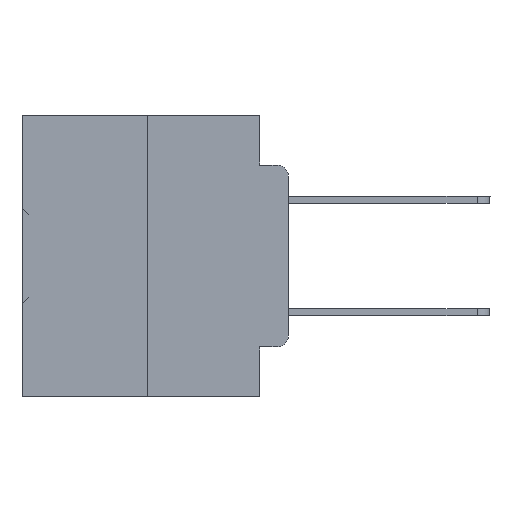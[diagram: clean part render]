
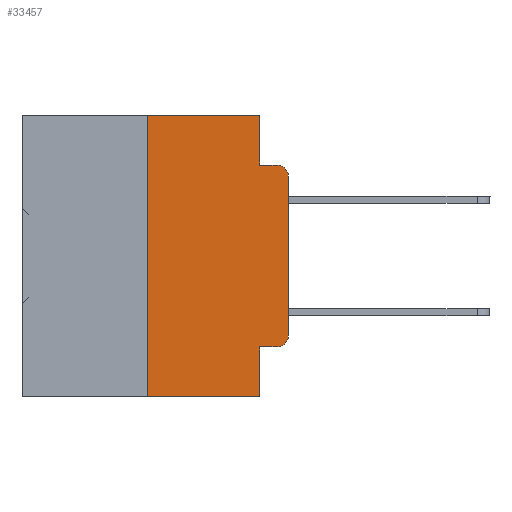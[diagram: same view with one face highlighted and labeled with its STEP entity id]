
A CAD part, left-side view. The second image highlights one B-rep face of the part: STEP entity #33457.
In plain terms, the highlighted planar face has unit normal (-1, 0, 0).
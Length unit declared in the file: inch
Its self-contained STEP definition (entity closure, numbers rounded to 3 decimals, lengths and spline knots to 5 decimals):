
#88 = CARTESIAN_POINT ( 'NONE',  ( 0., 0.02, -0.3915 ) ) ;
#1342 = ORIENTED_EDGE ( 'NONE', *, *, #35961, .T. ) ;
#1684 = CIRCLE ( 'NONE', #11143, 0.02 ) ;
#2079 = ORIENTED_EDGE ( 'NONE', *, *, #12284, .F. ) ;
#2376 = DIRECTION ( 'NONE',  ( 0., 0., 1. ) ) ;
#2978 = ORIENTED_EDGE ( 'NONE', *, *, #35231, .T. ) ;
#3258 = DIRECTION ( 'NONE',  ( 0., -1., 0. ) ) ;
#3757 = ORIENTED_EDGE ( 'NONE', *, *, #28549, .T. ) ;
#3790 = CARTESIAN_POINT ( 'NONE',  ( 0., 0.02, -0.1085 ) ) ;
#4803 = VECTOR ( 'NONE', #38339, 39.37008 ) ;
#5475 = CARTESIAN_POINT ( 'NONE',  ( 0., 0.051, 0. ) ) ;
#5588 = VERTEX_POINT ( 'NONE', #29817 ) ;
#5897 = VERTEX_POINT ( 'NONE', #31747 ) ;
#6473 = EDGE_CURVE ( 'NONE', #5588, #16402, #15289, .T. ) ;
#6574 = VERTEX_POINT ( 'NONE', #9581 ) ;
#6600 = LINE ( 'NONE', #30233, #21007 ) ;
#6768 = CARTESIAN_POINT ( 'NONE',  ( 0., 0.25, 0. ) ) ;
#6769 = VECTOR ( 'NONE', #21133, 39.37008 ) ;
#7254 = AXIS2_PLACEMENT_3D ( 'NONE', #20792, #32813, #12151 ) ;
#8022 = VECTOR ( 'NONE', #2376, 39.37008 ) ;
#8224 = VERTEX_POINT ( 'NONE', #24712 ) ;
#9144 = CARTESIAN_POINT ( 'NONE',  ( 0., 0.051, -0.4115 ) ) ;
#9257 = LINE ( 'NONE', #21049, #28748 ) ;
#9489 = DIRECTION ( 'NONE',  ( 0., 0., -1. ) ) ;
#9581 = CARTESIAN_POINT ( 'NONE',  ( 0., 0.02, -0.4115 ) ) ;
#9919 = LINE ( 'NONE', #6768, #32879 ) ;
#11143 = AXIS2_PLACEMENT_3D ( 'NONE', #3790, #12254, #9489 ) ;
#11193 = EDGE_CURVE ( 'NONE', #8224, #28474, #9919, .T. ) ;
#11759 = LINE ( 'NONE', #5475, #17265 ) ;
#12151 = DIRECTION ( 'NONE',  ( 0., 0., -1. ) ) ;
#12228 = ORIENTED_EDGE ( 'NONE', *, *, #6473, .F. ) ;
#12254 = DIRECTION ( 'NONE',  ( -1., 0., 0. ) ) ;
#12284 = EDGE_CURVE ( 'NONE', #23828, #20563, #11759, .T. ) ;
#12286 = DIRECTION ( 'NONE',  ( -1., 0., 0. ) ) ;
#12354 = CARTESIAN_POINT ( 'NONE',  ( 0., 0.051, 0. ) ) ;
#12408 = DIRECTION ( 'NONE',  ( 0., -1., 0. ) ) ;
#14841 = CARTESIAN_POINT ( 'NONE',  ( 0., 0.25, 0. ) ) ;
#14842 = LINE ( 'NONE', #9144, #6769 ) ;
#15289 = LINE ( 'NONE', #12354, #19162 ) ;
#15735 = EDGE_LOOP ( 'NONE', ( #28752, #2978, #20621, #2079, #34909, #27497, #1342, #12228, #30857, #3757 ) ) ;
#15802 = DIRECTION ( 'NONE',  ( 0., 0., 1. ) ) ;
#16402 = VERTEX_POINT ( 'NONE', #34212 ) ;
#17099 = LINE ( 'NONE', #26152, #4803 ) ;
#17265 = VECTOR ( 'NONE', #17465, 39.37008 ) ;
#17465 = DIRECTION ( 'NONE',  ( 0., 0., -1. ) ) ;
#17631 = CIRCLE ( 'NONE', #30202, 0.02 ) ;
#18245 = DIRECTION ( 'NONE',  ( 0., 0., -1. ) ) ;
#19144 = CARTESIAN_POINT ( 'NONE',  ( 0., 0.051, 0. ) ) ;
#19162 = VECTOR ( 'NONE', #18245, 39.37008 ) ;
#20358 = EDGE_CURVE ( 'NONE', #20563, #5897, #6600, .T. ) ;
#20563 = VERTEX_POINT ( 'NONE', #31199 ) ;
#20621 = ORIENTED_EDGE ( 'NONE', *, *, #20358, .F. ) ;
#20792 = CARTESIAN_POINT ( 'NONE',  ( 0., 0.473, 0. ) ) ;
#21007 = VECTOR ( 'NONE', #3258, 39.37008 ) ;
#21049 = CARTESIAN_POINT ( 'NONE',  ( 0., 0.473, 0. ) ) ;
#21131 = DIRECTION ( 'NONE',  ( 0., 0., -1. ) ) ;
#21133 = DIRECTION ( 'NONE',  ( 0., -1., 0. ) ) ;
#23156 = CARTESIAN_POINT ( 'NONE',  ( 0., 0., -0.1085 ) ) ;
#23620 = CARTESIAN_POINT ( 'NONE',  ( 0., 0., 0. ) ) ;
#23624 = EDGE_CURVE ( 'NONE', #5588, #6574, #14842, .T. ) ;
#23815 = LINE ( 'NONE', #23620, #8022 ) ;
#23828 = VERTEX_POINT ( 'NONE', #19144 ) ;
#24712 = CARTESIAN_POINT ( 'NONE',  ( 0., 0.25, -0.5 ) ) ;
#26152 = CARTESIAN_POINT ( 'NONE',  ( 0., 0.473, -0.5 ) ) ;
#26919 = PLANE ( 'NONE',  #7254 ) ;
#27497 = ORIENTED_EDGE ( 'NONE', *, *, #11193, .F. ) ;
#28474 = VERTEX_POINT ( 'NONE', #14841 ) ;
#28549 = EDGE_CURVE ( 'NONE', #6574, #29519, #17631, .T. ) ;
#28748 = VECTOR ( 'NONE', #12408, 39.37008 ) ;
#28752 = ORIENTED_EDGE ( 'NONE', *, *, #35574, .T. ) ;
#29440 = CARTESIAN_POINT ( 'NONE',  ( 0., 0., -0.3915 ) ) ;
#29519 = VERTEX_POINT ( 'NONE', #29440 ) ;
#29817 = CARTESIAN_POINT ( 'NONE',  ( 0., 0.051, -0.4115 ) ) ;
#30202 = AXIS2_PLACEMENT_3D ( 'NONE', #88, #12286, #21131 ) ;
#30233 = CARTESIAN_POINT ( 'NONE',  ( 0., 0.051, -0.0885 ) ) ;
#30857 = ORIENTED_EDGE ( 'NONE', *, *, #23624, .T. ) ;
#31199 = CARTESIAN_POINT ( 'NONE',  ( 0., 0.051, -0.0885 ) ) ;
#31747 = CARTESIAN_POINT ( 'NONE',  ( 0., 0.02, -0.0885 ) ) ;
#32108 = VERTEX_POINT ( 'NONE', #23156 ) ;
#32813 = DIRECTION ( 'NONE',  ( 1., 0., 0. ) ) ;
#32879 = VECTOR ( 'NONE', #15802, 39.37008 ) ;
#33457 = ADVANCED_FACE ( 'NONE', ( #33596 ), #26919, .F. ) ;
#33596 = FACE_OUTER_BOUND ( 'NONE', #15735, .T. ) ;
#34212 = CARTESIAN_POINT ( 'NONE',  ( 0., 0.051, -0.5 ) ) ;
#34909 = ORIENTED_EDGE ( 'NONE', *, *, #35665, .F. ) ;
#35231 = EDGE_CURVE ( 'NONE', #32108, #5897, #1684, .T. ) ;
#35574 = EDGE_CURVE ( 'NONE', #29519, #32108, #23815, .T. ) ;
#35665 = EDGE_CURVE ( 'NONE', #28474, #23828, #9257, .T. ) ;
#35961 = EDGE_CURVE ( 'NONE', #8224, #16402, #17099, .T. ) ;
#38339 = DIRECTION ( 'NONE',  ( 0., -1., 0. ) ) ;
